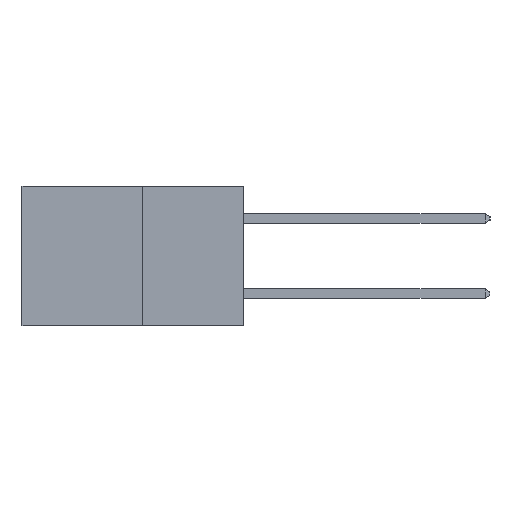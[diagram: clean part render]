
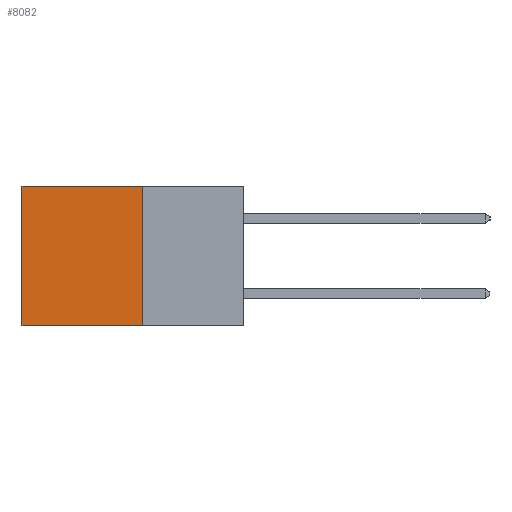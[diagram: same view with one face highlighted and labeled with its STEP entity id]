
A CAD part, left-side view. The second image highlights one B-rep face of the part: STEP entity #8082.
In plain terms, the highlighted planar face has unit normal (-1, 0, 0).
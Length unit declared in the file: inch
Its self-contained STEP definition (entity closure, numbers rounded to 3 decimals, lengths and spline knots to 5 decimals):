
#534 = ORIENTED_EDGE ( 'NONE', *, *, #1820, .T. ) ;
#627 = ORIENTED_EDGE ( 'NONE', *, *, #5751, .F. ) ;
#676 = VECTOR ( 'NONE', #5344, 39.37008 ) ;
#1494 = AXIS2_PLACEMENT_3D ( 'NONE', #7413, #3044, #8129 ) ;
#1820 = EDGE_CURVE ( 'NONE', #3222, #8882, #8971, .T. ) ;
#2226 = CARTESIAN_POINT ( 'NONE',  ( 0.277, 0.27, -0.37 ) ) ;
#2565 = EDGE_LOOP ( 'NONE', ( #534, #6430, #627, #4579 ) ) ;
#3044 = DIRECTION ( 'NONE',  ( 1., 0., 0. ) ) ;
#3222 = VERTEX_POINT ( 'NONE', #3808 ) ;
#3808 = CARTESIAN_POINT ( 'NONE',  ( 0.277, 0.59, 0. ) ) ;
#4262 = FACE_OUTER_BOUND ( 'NONE', #2565, .T. ) ;
#4390 = VERTEX_POINT ( 'NONE', #8669 ) ;
#4411 = VERTEX_POINT ( 'NONE', #5257 ) ;
#4579 = ORIENTED_EDGE ( 'NONE', *, *, #5793, .T. ) ;
#5060 = LINE ( 'NONE', #5658, #5545 ) ;
#5203 = PLANE ( 'NONE',  #1494 ) ;
#5257 = CARTESIAN_POINT ( 'NONE',  ( 0.277, 0.27, 0. ) ) ;
#5344 = DIRECTION ( 'NONE',  ( 0., 1., 0. ) ) ;
#5457 = CARTESIAN_POINT ( 'NONE',  ( 0.277, 0.27, 0. ) ) ;
#5545 = VECTOR ( 'NONE', #5712, 39.37008 ) ;
#5651 = CARTESIAN_POINT ( 'NONE',  ( 0.277, 0.59, -0.37 ) ) ;
#5658 = CARTESIAN_POINT ( 'NONE',  ( 0.277, 0.27, -0.37 ) ) ;
#5712 = DIRECTION ( 'NONE',  ( 0., 0., -1. ) ) ;
#5751 = EDGE_CURVE ( 'NONE', #4411, #4390, #5060, .T. ) ;
#5793 = EDGE_CURVE ( 'NONE', #4411, #3222, #8479, .T. ) ;
#6430 = ORIENTED_EDGE ( 'NONE', *, *, #8502, .F. ) ;
#6706 = DIRECTION ( 'NONE',  ( 0., 0., -1. ) ) ;
#6713 = CARTESIAN_POINT ( 'NONE',  ( 0.277, 0.59, -0.37 ) ) ;
#7049 = VECTOR ( 'NONE', #6706, 39.37008 ) ;
#7356 = DIRECTION ( 'NONE',  ( 0., 1., 0. ) ) ;
#7413 = CARTESIAN_POINT ( 'NONE',  ( 0.277, 0.27, -0.37 ) ) ;
#7441 = VECTOR ( 'NONE', #7356, 39.37008 ) ;
#8082 = ADVANCED_FACE ( 'NONE', ( #4262 ), #5203, .F. ) ;
#8129 = DIRECTION ( 'NONE',  ( 0., 0., -1. ) ) ;
#8479 = LINE ( 'NONE', #5457, #676 ) ;
#8502 = EDGE_CURVE ( 'NONE', #4390, #8882, #9314, .T. ) ;
#8669 = CARTESIAN_POINT ( 'NONE',  ( 0.277, 0.27, -0.37 ) ) ;
#8882 = VERTEX_POINT ( 'NONE', #5651 ) ;
#8971 = LINE ( 'NONE', #6713, #7049 ) ;
#9314 = LINE ( 'NONE', #2226, #7441 ) ;
